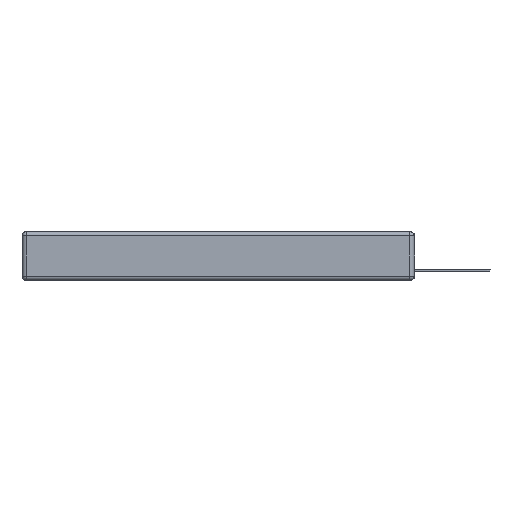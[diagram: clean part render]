
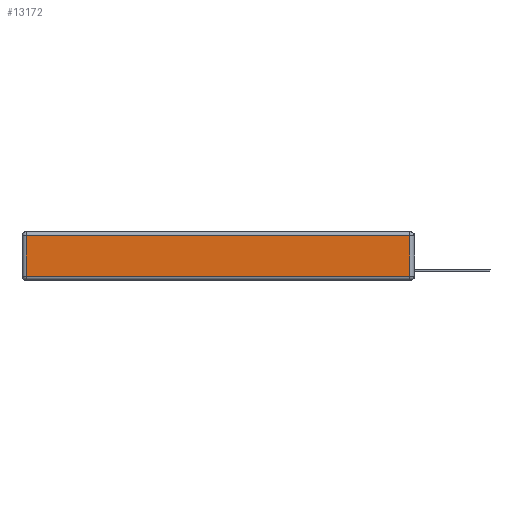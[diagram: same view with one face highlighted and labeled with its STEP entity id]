
A CAD part, left-side view. The second image highlights one B-rep face of the part: STEP entity #13172.
In plain terms, the highlighted planar face has unit normal (-1, 0, 0).
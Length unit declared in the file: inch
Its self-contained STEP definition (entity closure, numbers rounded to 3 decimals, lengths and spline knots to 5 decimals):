
#1168 = PLANE ( 'NONE',  #14783 ) ;
#1554 = EDGE_CURVE ( 'NONE', #7332, #11924, #15108, .T. ) ;
#2255 = FACE_OUTER_BOUND ( 'NONE', #13405, .T. ) ;
#2483 = CARTESIAN_POINT ( 'NONE',  ( 0., 0., -0.313 ) ) ;
#2609 = CARTESIAN_POINT ( 'NONE',  ( 0., 2.75, -0.03 ) ) ;
#4361 = CARTESIAN_POINT ( 'NONE',  ( 0., 0., -0.343 ) ) ;
#4974 = ORIENTED_EDGE ( 'NONE', *, *, #12577, .T. ) ;
#5949 = DIRECTION ( 'NONE',  ( 0., 0., 1. ) ) ;
#6304 = VERTEX_POINT ( 'NONE', #8762 ) ;
#6334 = ORIENTED_EDGE ( 'NONE', *, *, #10624, .T. ) ;
#6464 = ORIENTED_EDGE ( 'NONE', *, *, #14796, .T. ) ;
#7332 = VERTEX_POINT ( 'NONE', #8946 ) ;
#8374 = CARTESIAN_POINT ( 'NONE',  ( 0., 2.72, -0.03 ) ) ;
#8762 = CARTESIAN_POINT ( 'NONE',  ( 0., 0.03, -0.03 ) ) ;
#8946 = CARTESIAN_POINT ( 'NONE',  ( 0., 2.72, -0.313 ) ) ;
#9132 = VECTOR ( 'NONE', #9389, 39.37008 ) ;
#9389 = DIRECTION ( 'NONE',  ( 0., 0., 1. ) ) ;
#9503 = VERTEX_POINT ( 'NONE', #8374 ) ;
#9513 = LINE ( 'NONE', #17136, #16649 ) ;
#10099 = LINE ( 'NONE', #2609, #17725 ) ;
#10347 = DIRECTION ( 'NONE',  ( 0., 1., 0. ) ) ;
#10624 = EDGE_CURVE ( 'NONE', #11924, #6304, #16755, .T. ) ;
#11924 = VERTEX_POINT ( 'NONE', #13691 ) ;
#12577 = EDGE_CURVE ( 'NONE', #6304, #9503, #10099, .T. ) ;
#13172 = ADVANCED_FACE ( 'NONE', ( #2255 ), #1168, .T. ) ;
#13405 = EDGE_LOOP ( 'NONE', ( #15780, #6334, #4974, #6464 ) ) ;
#13691 = CARTESIAN_POINT ( 'NONE',  ( 0., 0.03, -0.313 ) ) ;
#14426 = DIRECTION ( 'NONE',  ( 0., -1., 0. ) ) ;
#14783 = AXIS2_PLACEMENT_3D ( 'NONE', #4361, #16389, #5949 ) ;
#14796 = EDGE_CURVE ( 'NONE', #9503, #7332, #9513, .T. ) ;
#15108 = LINE ( 'NONE', #2483, #19596 ) ;
#15671 = DIRECTION ( 'NONE',  ( 0., 0., -1. ) ) ;
#15780 = ORIENTED_EDGE ( 'NONE', *, *, #1554, .T. ) ;
#16389 = DIRECTION ( 'NONE',  ( -1., 0., 0. ) ) ;
#16649 = VECTOR ( 'NONE', #15671, 39.37008 ) ;
#16755 = LINE ( 'NONE', #18487, #9132 ) ;
#17136 = CARTESIAN_POINT ( 'NONE',  ( 0., 2.72, -0.343 ) ) ;
#17725 = VECTOR ( 'NONE', #10347, 39.37008 ) ;
#18487 = CARTESIAN_POINT ( 'NONE',  ( 0., 0.03, -0.343 ) ) ;
#19596 = VECTOR ( 'NONE', #14426, 39.37008 ) ;
